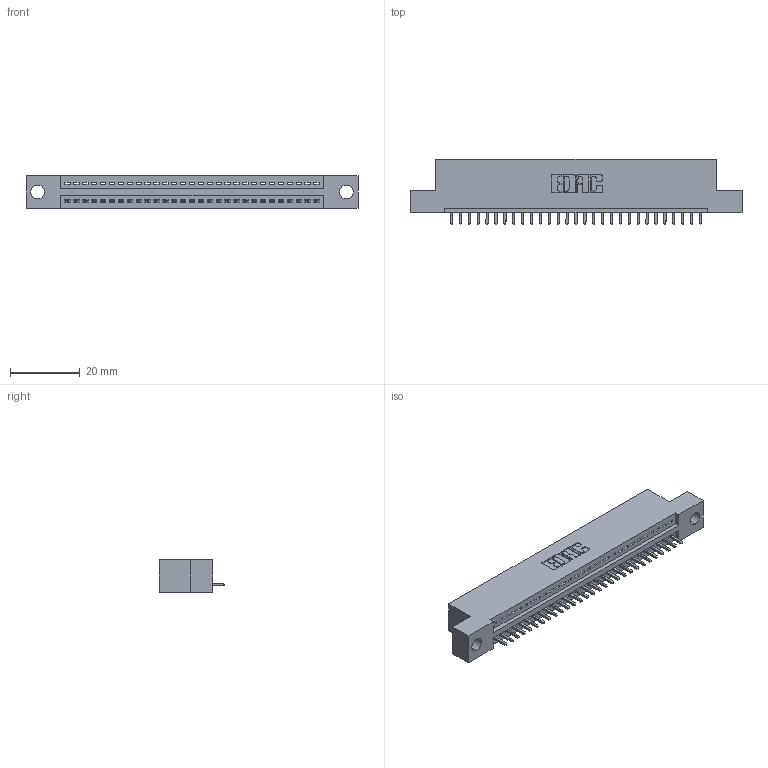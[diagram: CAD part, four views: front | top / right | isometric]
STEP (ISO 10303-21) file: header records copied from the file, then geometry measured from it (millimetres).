
FILE_DESCRIPTION (( 'STEP AP203' ), '1' );
FILE_NAME ('395-029-521-104.STEP', '2021-05-31T14:41:48', ( '' ), ( '' ), 'SwSTEP 2.0', 'SolidWorks 2020', '' );
FILE_SCHEMA (( 'CONFIG_CONTROL_DESIGN' ));
Length unit declared in the file: inch
Products named in the file (3): 345-292-001_345-293-121; 345 Part_Flush Mounting Lugs - 0.156 Dia-TI; 395-029-521-104
Assembly tree (30 placements, depth 2):
  395-029-521-104
    345 Part_Flush Mounting Lugs - 0.156 Dia-TI
    345-292-001_345-293-121  x29
Bounding box: 94.87 x 18.72 x 9.4 mm (x, y, z)
Volume: 8715.8 mm3; surface area: 10925.6 mm2
Topology: 30 solids, 30 shells, 1822 faces, 5481 edges, 3614 vertices
Faces by surface type: plane 1254, cylinder 568
Entity records: 24013 total; most frequent: CARTESIAN_POINT 4169, ORIENTED_EDGE 4130, DIRECTION 3659, EDGE_CURVE 2065, LINE 1817, VECTOR 1817, VERTEX_POINT 1374, AXIS2_PLACEMENT_3D 921
